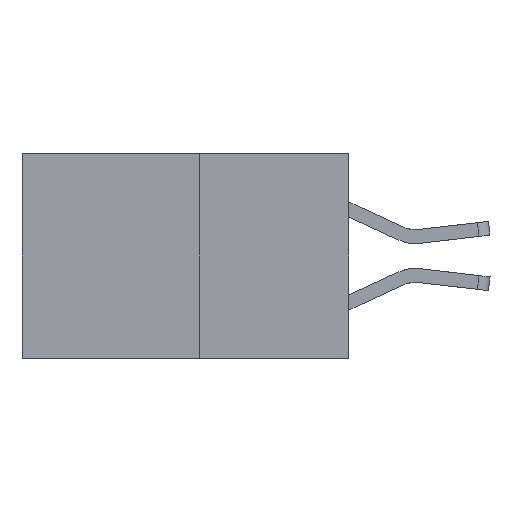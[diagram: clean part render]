
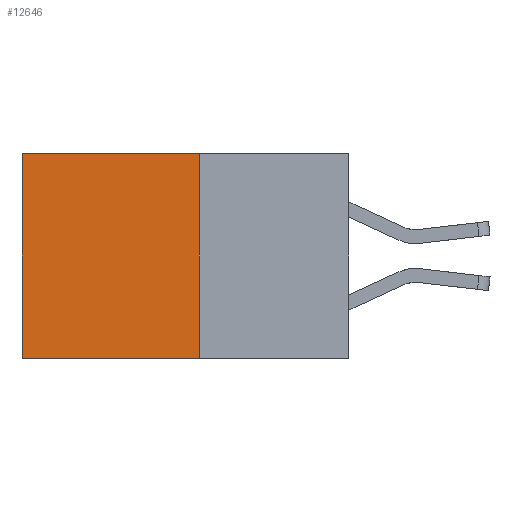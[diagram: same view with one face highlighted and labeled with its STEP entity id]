
A CAD part, left-side view. The second image highlights one B-rep face of the part: STEP entity #12646.
In plain terms, the highlighted planar face has unit normal (-1, 0, 0).
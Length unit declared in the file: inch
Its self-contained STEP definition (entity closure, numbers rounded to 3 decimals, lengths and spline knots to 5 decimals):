
#286 = LINE ( 'NONE', #4674, #2493 ) ;
#325 = VECTOR ( 'NONE', #13316, 39.37008 ) ;
#1050 = ORIENTED_EDGE ( 'NONE', *, *, #2038, .F. ) ;
#1073 = CARTESIAN_POINT ( 'NONE',  ( 0.277, 0.27, -0.37 ) ) ;
#1383 = CARTESIAN_POINT ( 'NONE',  ( 0.277, 0.59, -0.37 ) ) ;
#1423 = PLANE ( 'NONE',  #9935 ) ;
#2038 = EDGE_CURVE ( 'NONE', #7606, #5234, #286, .T. ) ;
#2493 = VECTOR ( 'NONE', #4591, 39.37008 ) ;
#2593 = CARTESIAN_POINT ( 'NONE',  ( 0.277, 0.59, -0.37 ) ) ;
#2612 = EDGE_CURVE ( 'NONE', #5234, #11142, #4260, .T. ) ;
#3250 = ORIENTED_EDGE ( 'NONE', *, *, #2612, .F. ) ;
#3908 = DIRECTION ( 'NONE',  ( 0., 1., 0. ) ) ;
#4222 = CARTESIAN_POINT ( 'NONE',  ( 0.277, 0.27, -0.37 ) ) ;
#4260 = LINE ( 'NONE', #4222, #9807 ) ;
#4591 = DIRECTION ( 'NONE',  ( 0., 0., -1. ) ) ;
#4620 = CARTESIAN_POINT ( 'NONE',  ( 0.277, 0.27, -0.37 ) ) ;
#4674 = CARTESIAN_POINT ( 'NONE',  ( 0.277, 0.27, -0.37 ) ) ;
#4982 = VERTEX_POINT ( 'NONE', #5436 ) ;
#5234 = VERTEX_POINT ( 'NONE', #1073 ) ;
#5436 = CARTESIAN_POINT ( 'NONE',  ( 0.277, 0.59, 0. ) ) ;
#5498 = DIRECTION ( 'NONE',  ( 0., 1., 0. ) ) ;
#5749 = DIRECTION ( 'NONE',  ( 0., 0., -1. ) ) ;
#6784 = ORIENTED_EDGE ( 'NONE', *, *, #8995, .T. ) ;
#7606 = VERTEX_POINT ( 'NONE', #10573 ) ;
#8327 = ORIENTED_EDGE ( 'NONE', *, *, #10411, .T. ) ;
#8926 = FACE_OUTER_BOUND ( 'NONE', #9428, .T. ) ;
#8995 = EDGE_CURVE ( 'NONE', #7606, #4982, #9034, .T. ) ;
#9034 = LINE ( 'NONE', #12088, #11952 ) ;
#9428 = EDGE_LOOP ( 'NONE', ( #8327, #3250, #1050, #6784 ) ) ;
#9807 = VECTOR ( 'NONE', #3908, 39.37008 ) ;
#9935 = AXIS2_PLACEMENT_3D ( 'NONE', #4620, #12341, #5749 ) ;
#10411 = EDGE_CURVE ( 'NONE', #4982, #11142, #11591, .T. ) ;
#10573 = CARTESIAN_POINT ( 'NONE',  ( 0.277, 0.27, 0. ) ) ;
#11142 = VERTEX_POINT ( 'NONE', #2593 ) ;
#11591 = LINE ( 'NONE', #1383, #325 ) ;
#11952 = VECTOR ( 'NONE', #5498, 39.37008 ) ;
#12088 = CARTESIAN_POINT ( 'NONE',  ( 0.277, 0.27, 0. ) ) ;
#12341 = DIRECTION ( 'NONE',  ( 1., 0., 0. ) ) ;
#12646 = ADVANCED_FACE ( 'NONE', ( #8926 ), #1423, .F. ) ;
#13316 = DIRECTION ( 'NONE',  ( 0., 0., -1. ) ) ;
